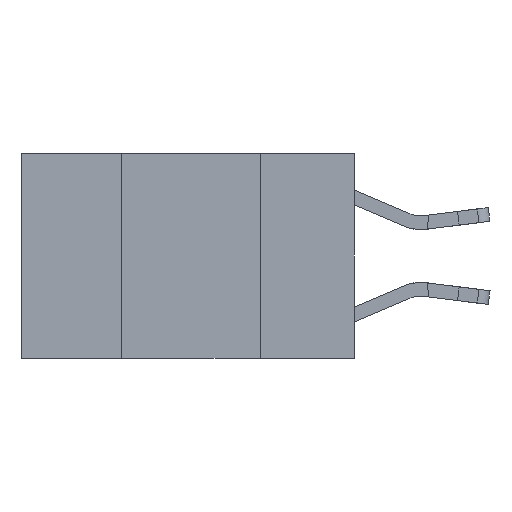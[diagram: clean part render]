
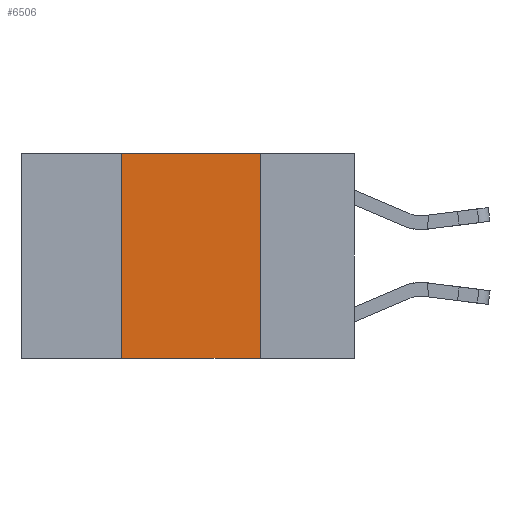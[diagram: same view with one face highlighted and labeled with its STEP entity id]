
A CAD part, left-side view. The second image highlights one B-rep face of the part: STEP entity #6506.
In plain terms, the highlighted planar face has unit normal (-1, 0, 0).
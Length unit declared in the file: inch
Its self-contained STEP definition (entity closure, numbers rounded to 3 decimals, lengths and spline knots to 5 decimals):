
#210 = VERTEX_POINT ( 'NONE', #10409 ) ;
#342 = CARTESIAN_POINT ( 'NONE',  ( 0., 0.6, 0. ) ) ;
#653 = DIRECTION ( 'NONE',  ( 0., -1., 0. ) ) ;
#1245 = PLANE ( 'NONE',  #7561 ) ;
#1544 = VECTOR ( 'NONE', #18405, 39.37008 ) ;
#1667 = EDGE_LOOP ( 'NONE', ( #8112, #8563, #16159, #5617 ) ) ;
#2692 = CARTESIAN_POINT ( 'NONE',  ( 0., 0.6, 0. ) ) ;
#3974 = VERTEX_POINT ( 'NONE', #13698 ) ;
#5617 = ORIENTED_EDGE ( 'NONE', *, *, #13323, .T. ) ;
#6506 = ADVANCED_FACE ( 'NONE', ( #13976 ), #1245, .F. ) ;
#7011 = DIRECTION ( 'NONE',  ( 0., 0., -1. ) ) ;
#7561 = AXIS2_PLACEMENT_3D ( 'NONE', #2692, #15613, #7011 ) ;
#7818 = LINE ( 'NONE', #10762, #15406 ) ;
#8112 = ORIENTED_EDGE ( 'NONE', *, *, #12373, .F. ) ;
#8457 = CARTESIAN_POINT ( 'NONE',  ( 0., 0.17, 0. ) ) ;
#8563 = ORIENTED_EDGE ( 'NONE', *, *, #8745, .F. ) ;
#8745 = EDGE_CURVE ( 'NONE', #210, #3974, #8995, .T. ) ;
#8901 = VERTEX_POINT ( 'NONE', #17430 ) ;
#8995 = LINE ( 'NONE', #342, #13262 ) ;
#10409 = CARTESIAN_POINT ( 'NONE',  ( 0., 0.42, 0. ) ) ;
#10424 = EDGE_CURVE ( 'NONE', #8901, #210, #13759, .T. ) ;
#10762 = CARTESIAN_POINT ( 'NONE',  ( 0., 0.6, -0.37 ) ) ;
#11846 = DIRECTION ( 'NONE',  ( 0., -1., 0. ) ) ;
#12373 = EDGE_CURVE ( 'NONE', #3974, #13799, #16361, .T. ) ;
#13262 = VECTOR ( 'NONE', #11846, 39.37008 ) ;
#13323 = EDGE_CURVE ( 'NONE', #8901, #13799, #7818, .T. ) ;
#13337 = VECTOR ( 'NONE', #18148, 39.37008 ) ;
#13698 = CARTESIAN_POINT ( 'NONE',  ( 0., 0.17, 0. ) ) ;
#13759 = LINE ( 'NONE', #16748, #13337 ) ;
#13799 = VERTEX_POINT ( 'NONE', #14530 ) ;
#13976 = FACE_OUTER_BOUND ( 'NONE', #1667, .T. ) ;
#14530 = CARTESIAN_POINT ( 'NONE',  ( 0., 0.17, -0.37 ) ) ;
#15406 = VECTOR ( 'NONE', #653, 39.37008 ) ;
#15613 = DIRECTION ( 'NONE',  ( 1., 0., 0. ) ) ;
#16159 = ORIENTED_EDGE ( 'NONE', *, *, #10424, .F. ) ;
#16361 = LINE ( 'NONE', #8457, #1544 ) ;
#16748 = CARTESIAN_POINT ( 'NONE',  ( 0., 0.42, 0. ) ) ;
#17430 = CARTESIAN_POINT ( 'NONE',  ( 0., 0.42, -0.37 ) ) ;
#18148 = DIRECTION ( 'NONE',  ( 0., 0., 1. ) ) ;
#18405 = DIRECTION ( 'NONE',  ( 0., 0., -1. ) ) ;
